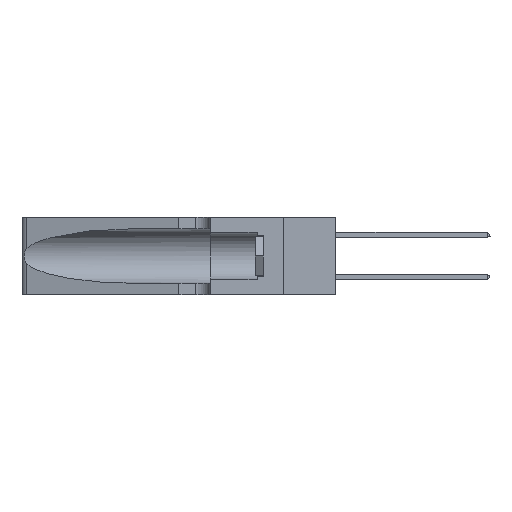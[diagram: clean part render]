
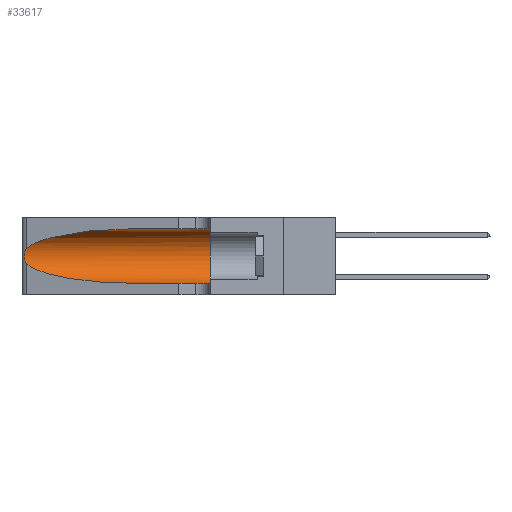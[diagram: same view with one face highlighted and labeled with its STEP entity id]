
A CAD part, left-side view. The second image highlights one B-rep face of the part: STEP entity #33617.
In plain terms, the highlighted cylindrical face has radius 3.308 mm (diameter 6.617 mm), a partial arc.
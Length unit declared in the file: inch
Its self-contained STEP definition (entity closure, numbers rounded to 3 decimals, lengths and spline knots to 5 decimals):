
#94 = EDGE_CURVE ( 'NONE', #23279, #14134, #28625, .T. ) ;
#540 = LINE ( 'NONE', #10392, #43192 ) ;
#806 = CARTESIAN_POINT ( 'NONE',  ( 0.18966, 0.96281, 0.05475 ) ) ;
#909 = VERTEX_POINT ( 'NONE', #44317 ) ;
#1113 = CARTESIAN_POINT ( 'NONE',  ( 0.25555, 1.22994, 0.2215 ) ) ;
#1264 = CARTESIAN_POINT ( 'NONE',  ( 0.25639, 1.23186, 0.15144 ) ) ;
#1522 = DIRECTION ( 'NONE',  ( 0., 0., 1. ) ) ;
#1799 = CARTESIAN_POINT ( 'NONE',  ( 0.1305, 0.72297, 0.31525 ) ) ;
#3148 = CARTESIAN_POINT ( 'NONE',  ( 0.25487, 1.22718, 0.22369 ) ) ;
#3179 =( BOUNDED_CURVE ( )  B_SPLINE_CURVE ( 3, ( #42148, #21525, #806, #25006 ),
 .UNSPECIFIED., .F., .F. ) 
 B_SPLINE_CURVE_WITH_KNOTS ( ( 4, 4 ),
 ( 3.44316, 4.71239 ),
 .UNSPECIFIED. ) 
 CURVE ( )  GEOMETRIC_REPRESENTATION_ITEM ( )  RATIONAL_B_SPLINE_CURVE ( ( 1., 0.87, 0.87, 1. ) ) 
 REPRESENTATION_ITEM ( '' )  );
#3768 = ORIENTED_EDGE ( 'NONE', *, *, #24122, .F. ) ;
#4270 = ORIENTED_EDGE ( 'NONE', *, *, #42832, .T. ) ;
#4744 = CARTESIAN_POINT ( 'NONE',  ( 0.25487, 1.22718, 0.14631 ) ) ;
#6004 = ORIENTED_EDGE ( 'NONE', *, *, #12424, .T. ) ;
#6620 = VERTEX_POINT ( 'NONE', #21350 ) ;
#7529 = CARTESIAN_POINT ( 'NONE',  ( 0.1305, 0.35, 0.31525 ) ) ;
#7721 = EDGE_CURVE ( 'NONE', #6620, #22636, #540, .T. ) ;
#8055 = CARTESIAN_POINT ( 'NONE',  ( 0.25639, 1.23184, 0.21858 ) ) ;
#8128 = CARTESIAN_POINT ( 'NONE',  ( 0.1305, 1.61858, 0.185 ) ) ;
#8754 = CARTESIAN_POINT ( 'NONE',  ( 0.18966, 0.96281, 0.31525 ) ) ;
#8802 = ORIENTED_EDGE ( 'NONE', *, *, #94, .T. ) ;
#10291 =( BOUNDED_CURVE ( )  B_SPLINE_CURVE ( 3, ( #1799, #8754, #36314, #15693 ),
 .UNSPECIFIED., .F., .F. ) 
 B_SPLINE_CURVE_WITH_KNOTS ( ( 4, 4 ),
 ( 1.5708, 2.84003 ),
 .UNSPECIFIED. ) 
 CURVE ( )  GEOMETRIC_REPRESENTATION_ITEM ( )  RATIONAL_B_SPLINE_CURVE ( ( 1., 0.87, 0.87, 1. ) ) 
 REPRESENTATION_ITEM ( '' )  );
#10392 = CARTESIAN_POINT ( 'NONE',  ( 0.1305, 1.61858, 0.31525 ) ) ;
#11557 = CARTESIAN_POINT ( 'NONE',  ( 0.25854, 1.2359, 0.20912 ) ) ;
#12424 = EDGE_CURVE ( 'NONE', #909, #23279, #3179, .T. ) ;
#14134 = VERTEX_POINT ( 'NONE', #17324 ) ;
#15023 = CARTESIAN_POINT ( 'NONE',  ( 0.26075, 1.23896, 0.19203 ) ) ;
#15158 = CYLINDRICAL_SURFACE ( 'NONE', #39709, 0.13025 ) ;
#15527 = AXIS2_PLACEMENT_3D ( 'NONE', #42848, #22243, #1522 ) ;
#15693 = CARTESIAN_POINT ( 'NONE',  ( 0.25487, 1.22718, 0.22369 ) ) ;
#17324 = CARTESIAN_POINT ( 'NONE',  ( 0.1305, 0.35, 0.05475 ) ) ;
#18190 = EDGE_LOOP ( 'NONE', ( #4270, #41842, #6004, #8802, #3768, #44044 ) ) ;
#18513 = CARTESIAN_POINT ( 'NONE',  ( 0.26017, 1.23833, 0.17102 ) ) ;
#21350 = CARTESIAN_POINT ( 'NONE',  ( 0.1305, 0.72297, 0.31525 ) ) ;
#21525 = CARTESIAN_POINT ( 'NONE',  ( 0.2373, 1.15595, 0.08982 ) ) ;
#21972 = CARTESIAN_POINT ( 'NONE',  ( 0.25789, 1.23486, 0.15765 ) ) ;
#22243 = DIRECTION ( 'NONE',  ( 0., 1., 0. ) ) ;
#22636 = VERTEX_POINT ( 'NONE', #7529 ) ;
#23020 = CARTESIAN_POINT ( 'NONE',  ( 0.1305, 1.61858, 0.05475 ) ) ;
#23279 = VERTEX_POINT ( 'NONE', #38388 ) ;
#24122 = EDGE_CURVE ( 'NONE', #22636, #14134, #24946, .T. ) ;
#24946 = CIRCLE ( 'NONE', #15527, 0.13025 ) ;
#25006 = CARTESIAN_POINT ( 'NONE',  ( 0.1305, 0.72297, 0.05475 ) ) ;
#25295 = CARTESIAN_POINT ( 'NONE',  ( 0.25487, 1.22718, 0.22369 ) ) ;
#25450 = CARTESIAN_POINT ( 'NONE',  ( 0.25555, 1.22993, 0.14849 ) ) ;
#28625 = LINE ( 'NONE', #23020, #37739 ) ;
#29455 = EDGE_CURVE ( 'NONE', #35343, #909, #38144, .T. ) ;
#32202 = CARTESIAN_POINT ( 'NONE',  ( 0.25787, 1.23484, 0.2124 ) ) ;
#32261 = DIRECTION ( 'NONE',  ( 0., 0., -1. ) ) ;
#33482 = FACE_OUTER_BOUND ( 'NONE', #18190, .T. ) ;
#33617 = ADVANCED_FACE ( 'NONE', ( #33482 ), #15158, .F. ) ;
#35343 = VERTEX_POINT ( 'NONE', #3148 ) ;
#35651 = CARTESIAN_POINT ( 'NONE',  ( 0.26018, 1.23835, 0.19895 ) ) ;
#36314 = CARTESIAN_POINT ( 'NONE',  ( 0.2373, 1.15595, 0.28018 ) ) ;
#37739 = VECTOR ( 'NONE', #40151, 39.37008 ) ;
#37960 = DIRECTION ( 'NONE',  ( 0., -1., 0. ) ) ;
#38144 = B_SPLINE_CURVE_WITH_KNOTS ( 'NONE', 3,
 ( #25295, #1113, #8055, #32202, #11557, #35651, #15023, #39120, #18513, #42588, #21972, #1264, #25450, #4744 ),
 .UNSPECIFIED., .F., .F.,
 ( 4, 2, 2, 2, 2, 2, 4 ),
 ( 0., 0.00027, 0.00053, 0.00107, 0.0016, 0.00187, 0.00214 ),
 .UNSPECIFIED. ) ;
#38388 = CARTESIAN_POINT ( 'NONE',  ( 0.1305, 0.72297, 0.05475 ) ) ;
#39120 = CARTESIAN_POINT ( 'NONE',  ( 0.26075, 1.23896, 0.178 ) ) ;
#39709 = AXIS2_PLACEMENT_3D ( 'NONE', #8128, #42352, #32261 ) ;
#40151 = DIRECTION ( 'NONE',  ( 0., -1., 0. ) ) ;
#41842 = ORIENTED_EDGE ( 'NONE', *, *, #29455, .T. ) ;
#42148 = CARTESIAN_POINT ( 'NONE',  ( 0.25487, 1.22718, 0.14631 ) ) ;
#42352 = DIRECTION ( 'NONE',  ( 0., -1., 0. ) ) ;
#42588 = CARTESIAN_POINT ( 'NONE',  ( 0.25856, 1.23593, 0.16098 ) ) ;
#42832 = EDGE_CURVE ( 'NONE', #6620, #35343, #10291, .T. ) ;
#42848 = CARTESIAN_POINT ( 'NONE',  ( 0.1305, 0.35, 0.185 ) ) ;
#43192 = VECTOR ( 'NONE', #37960, 39.37008 ) ;
#44044 = ORIENTED_EDGE ( 'NONE', *, *, #7721, .F. ) ;
#44317 = CARTESIAN_POINT ( 'NONE',  ( 0.25487, 1.22718, 0.14631 ) ) ;
